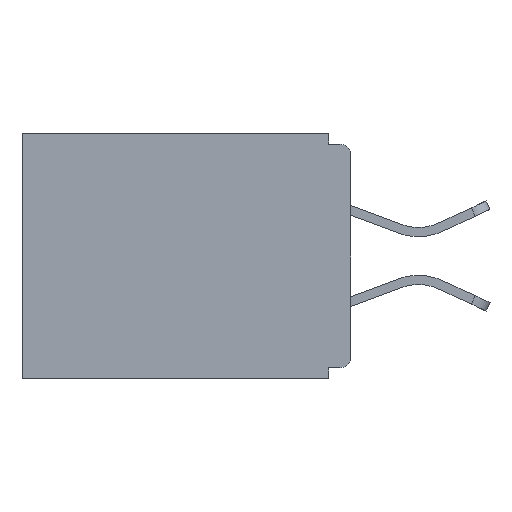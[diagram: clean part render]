
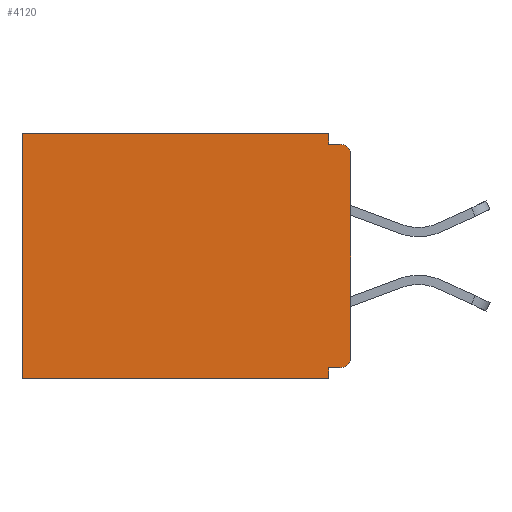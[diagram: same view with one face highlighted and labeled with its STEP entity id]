
A CAD part, left-side view. The second image highlights one B-rep face of the part: STEP entity #4120.
In plain terms, the highlighted planar face has unit normal (-1, 0, 0).
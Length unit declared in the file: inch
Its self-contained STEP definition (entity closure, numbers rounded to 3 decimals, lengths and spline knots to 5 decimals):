
#97 = FACE_OUTER_BOUND ( 'NONE', #2529, .T. ) ;
#441 = LINE ( 'NONE', #10510, #12625 ) ;
#793 = ORIENTED_EDGE ( 'NONE', *, *, #4534, .F. ) ;
#844 = CARTESIAN_POINT ( 'NONE',  ( 0.298, 0.46, 0. ) ) ;
#1063 = CIRCLE ( 'NONE', #8835, 0.015 ) ;
#1237 = EDGE_CURVE ( 'NONE', #9859, #12657, #441, .T. ) ;
#1301 = VERTEX_POINT ( 'NONE', #6046 ) ;
#1745 = EDGE_CURVE ( 'NONE', #16130, #16019, #3956, .T. ) ;
#2529 = EDGE_LOOP ( 'NONE', ( #11908, #17271, #18731, #5228, #16068, #16784, #3318, #793, #12062, #9273 ) ) ;
#2925 = CARTESIAN_POINT ( 'NONE',  ( 0.298, 0.015, -0.03 ) ) ;
#2928 = EDGE_CURVE ( 'NONE', #13561, #12657, #16614, .T. ) ;
#2929 = LINE ( 'NONE', #10419, #16538 ) ;
#3048 = DIRECTION ( 'NONE',  ( 1., 0., 0. ) ) ;
#3162 = DIRECTION ( 'NONE',  ( 0., 0., -1. ) ) ;
#3196 = CARTESIAN_POINT ( 'NONE',  ( 0.298, 0.031, -0.343 ) ) ;
#3210 = VERTEX_POINT ( 'NONE', #19289 ) ;
#3318 = ORIENTED_EDGE ( 'NONE', *, *, #12330, .F. ) ;
#3918 = LINE ( 'NONE', #4491, #6498 ) ;
#3956 = LINE ( 'NONE', #14474, #11921 ) ;
#4043 = VERTEX_POINT ( 'NONE', #5122 ) ;
#4120 = ADVANCED_FACE ( 'NONE', ( #97 ), #6731, .F. ) ;
#4175 = DIRECTION ( 'NONE',  ( 0., 0., -1. ) ) ;
#4491 = CARTESIAN_POINT ( 'NONE',  ( 0.298, 0.031, -0.343 ) ) ;
#4534 = EDGE_CURVE ( 'NONE', #13561, #1301, #2929, .T. ) ;
#4745 = DIRECTION ( 'NONE',  ( 0., 1., 0. ) ) ;
#5122 = CARTESIAN_POINT ( 'NONE',  ( 0.298, 0.031, -0.015 ) ) ;
#5228 = ORIENTED_EDGE ( 'NONE', *, *, #1745, .T. ) ;
#5357 = EDGE_CURVE ( 'NONE', #16130, #4043, #10153, .T. ) ;
#5786 = DIRECTION ( 'NONE',  ( -1., 0., 0. ) ) ;
#5850 = CARTESIAN_POINT ( 'NONE',  ( 0.298, 0.031, -0.343 ) ) ;
#6046 = CARTESIAN_POINT ( 'NONE',  ( 0.298, 0.031, -0.328 ) ) ;
#6060 = DIRECTION ( 'NONE',  ( 0., -1., 0. ) ) ;
#6498 = VECTOR ( 'NONE', #12063, 39.37008 ) ;
#6731 = PLANE ( 'NONE',  #17180 ) ;
#7211 = CARTESIAN_POINT ( 'NONE',  ( 0.298, 0.015, -0.015 ) ) ;
#7339 = DIRECTION ( 'NONE',  ( 0., 1., 0. ) ) ;
#7368 = DIRECTION ( 'NONE',  ( 0., 0., -1. ) ) ;
#7551 = DIRECTION ( 'NONE',  ( -1., 0., 0. ) ) ;
#8644 = VECTOR ( 'NONE', #4745, 39.37008 ) ;
#8835 = AXIS2_PLACEMENT_3D ( 'NONE', #2925, #5786, #4175 ) ;
#9099 = LINE ( 'NONE', #15043, #11219 ) ;
#9273 = ORIENTED_EDGE ( 'NONE', *, *, #1237, .F. ) ;
#9728 = CARTESIAN_POINT ( 'NONE',  ( 0.298, 0., 0. ) ) ;
#9815 = DIRECTION ( 'NONE',  ( 0., 1., 0. ) ) ;
#9859 = VERTEX_POINT ( 'NONE', #11113 ) ;
#10031 = DIRECTION ( 'NONE',  ( 0., 0., -1. ) ) ;
#10153 = LINE ( 'NONE', #5850, #19073 ) ;
#10419 = CARTESIAN_POINT ( 'NONE',  ( 0.298, 0., -0.328 ) ) ;
#10424 = CARTESIAN_POINT ( 'NONE',  ( 0.298, 0.46, 0. ) ) ;
#10510 = CARTESIAN_POINT ( 'NONE',  ( 0.298, 0., 0. ) ) ;
#10831 = EDGE_CURVE ( 'NONE', #16567, #3210, #14280, .T. ) ;
#10866 = CARTESIAN_POINT ( 'NONE',  ( 0.298, 0.015, -0.313 ) ) ;
#11113 = CARTESIAN_POINT ( 'NONE',  ( 0.298, 0., -0.03 ) ) ;
#11219 = VECTOR ( 'NONE', #6060, 39.37008 ) ;
#11750 = EDGE_CURVE ( 'NONE', #4043, #13040, #9099, .T. ) ;
#11908 = ORIENTED_EDGE ( 'NONE', *, *, #12486, .T. ) ;
#11921 = VECTOR ( 'NONE', #9815, 39.37008 ) ;
#12054 = EDGE_CURVE ( 'NONE', #16019, #3210, #12387, .T. ) ;
#12062 = ORIENTED_EDGE ( 'NONE', *, *, #2928, .T. ) ;
#12063 = DIRECTION ( 'NONE',  ( 0., 0., -1. ) ) ;
#12330 = EDGE_CURVE ( 'NONE', #1301, #16567, #3918, .T. ) ;
#12387 = LINE ( 'NONE', #844, #18057 ) ;
#12486 = EDGE_CURVE ( 'NONE', #9859, #13040, #1063, .T. ) ;
#12625 = VECTOR ( 'NONE', #3162, 39.37008 ) ;
#12657 = VERTEX_POINT ( 'NONE', #14233 ) ;
#13040 = VERTEX_POINT ( 'NONE', #7211 ) ;
#13438 = CARTESIAN_POINT ( 'NONE',  ( 0.298, 0., -0.343 ) ) ;
#13561 = VERTEX_POINT ( 'NONE', #17187 ) ;
#14233 = CARTESIAN_POINT ( 'NONE',  ( 0.298, 0., -0.313 ) ) ;
#14280 = LINE ( 'NONE', #13438, #8644 ) ;
#14474 = CARTESIAN_POINT ( 'NONE',  ( 0.298, 0., 0. ) ) ;
#15043 = CARTESIAN_POINT ( 'NONE',  ( 0.298, 0., -0.015 ) ) ;
#15622 = AXIS2_PLACEMENT_3D ( 'NONE', #10866, #7551, #7368 ) ;
#16019 = VERTEX_POINT ( 'NONE', #10424 ) ;
#16068 = ORIENTED_EDGE ( 'NONE', *, *, #12054, .T. ) ;
#16130 = VERTEX_POINT ( 'NONE', #16677 ) ;
#16538 = VECTOR ( 'NONE', #7339, 39.37008 ) ;
#16567 = VERTEX_POINT ( 'NONE', #3196 ) ;
#16614 = CIRCLE ( 'NONE', #15622, 0.015 ) ;
#16677 = CARTESIAN_POINT ( 'NONE',  ( 0.298, 0.031, 0. ) ) ;
#16784 = ORIENTED_EDGE ( 'NONE', *, *, #10831, .F. ) ;
#17180 = AXIS2_PLACEMENT_3D ( 'NONE', #9728, #3048, #17955 ) ;
#17187 = CARTESIAN_POINT ( 'NONE',  ( 0.298, 0.015, -0.328 ) ) ;
#17271 = ORIENTED_EDGE ( 'NONE', *, *, #11750, .F. ) ;
#17955 = DIRECTION ( 'NONE',  ( 0., 0., -1. ) ) ;
#18057 = VECTOR ( 'NONE', #10031, 39.37008 ) ;
#18731 = ORIENTED_EDGE ( 'NONE', *, *, #5357, .F. ) ;
#19073 = VECTOR ( 'NONE', #19379, 39.37008 ) ;
#19289 = CARTESIAN_POINT ( 'NONE',  ( 0.298, 0.46, -0.343 ) ) ;
#19379 = DIRECTION ( 'NONE',  ( 0., 0., -1. ) ) ;
